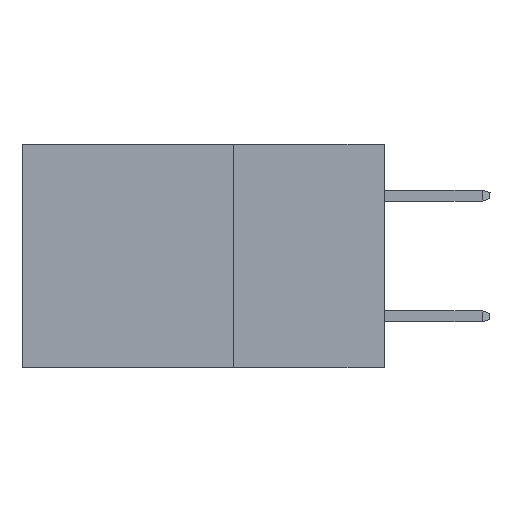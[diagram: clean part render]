
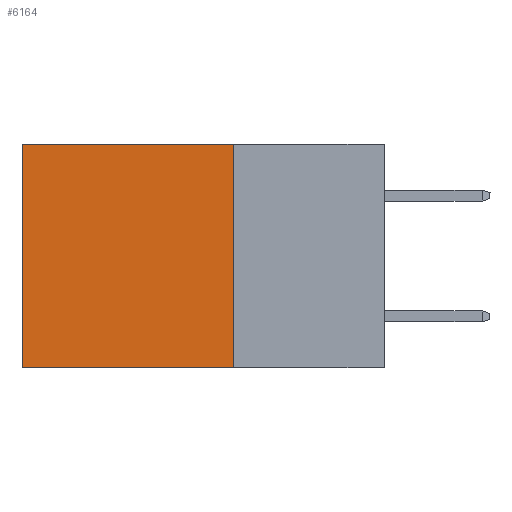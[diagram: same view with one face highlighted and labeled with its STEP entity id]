
A CAD part, left-side view. The second image highlights one B-rep face of the part: STEP entity #6164.
In plain terms, the highlighted planar face has unit normal (-1, 0, 0).
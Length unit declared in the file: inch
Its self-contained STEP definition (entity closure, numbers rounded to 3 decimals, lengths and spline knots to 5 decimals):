
#123 = EDGE_CURVE ( 'NONE', #22109, #328, #17010, .T. ) ;
#328 = VERTEX_POINT ( 'NONE', #18440 ) ;
#465 = DIRECTION ( 'NONE',  ( 0., 0., -1. ) ) ;
#717 = ORIENTED_EDGE ( 'NONE', *, *, #6820, .T. ) ;
#1364 = VERTEX_POINT ( 'NONE', #5905 ) ;
#1472 = EDGE_CURVE ( 'NONE', #1364, #22109, #12091, .T. ) ;
#4559 = ORIENTED_EDGE ( 'NONE', *, *, #123, .F. ) ;
#5905 = CARTESIAN_POINT ( 'NONE',  ( 0.298, 0.25, 0. ) ) ;
#6044 = CARTESIAN_POINT ( 'NONE',  ( 0.298, 0.25, -0.37 ) ) ;
#6164 = ADVANCED_FACE ( 'NONE', ( #22133 ), #16163, .F. ) ;
#6183 = DIRECTION ( 'NONE',  ( 0., 1., 0. ) ) ;
#6373 = DIRECTION ( 'NONE',  ( 0., 0., -1. ) ) ;
#6401 = DIRECTION ( 'NONE',  ( 0., 1., 0. ) ) ;
#6491 = CARTESIAN_POINT ( 'NONE',  ( 0.298, 0.25, 0. ) ) ;
#6820 = EDGE_CURVE ( 'NONE', #1364, #8676, #20206, .T. ) ;
#7930 = EDGE_CURVE ( 'NONE', #8676, #328, #10100, .T. ) ;
#8676 = VERTEX_POINT ( 'NONE', #9246 ) ;
#8745 = VECTOR ( 'NONE', #6373, 39.37008 ) ;
#9246 = CARTESIAN_POINT ( 'NONE',  ( 0.298, 0.6, 0. ) ) ;
#9337 = VECTOR ( 'NONE', #6183, 39.37008 ) ;
#9943 = EDGE_LOOP ( 'NONE', ( #10890, #4559, #16359, #717 ) ) ;
#10100 = LINE ( 'NONE', #16648, #8745 ) ;
#10747 = CARTESIAN_POINT ( 'NONE',  ( 0.298, 0.25, 0. ) ) ;
#10890 = ORIENTED_EDGE ( 'NONE', *, *, #7930, .T. ) ;
#11687 = CARTESIAN_POINT ( 'NONE',  ( 0.298, 0.25, -0.37 ) ) ;
#12091 = LINE ( 'NONE', #10747, #15874 ) ;
#15133 = AXIS2_PLACEMENT_3D ( 'NONE', #16238, #21469, #19592 ) ;
#15874 = VECTOR ( 'NONE', #465, 39.37008 ) ;
#16163 = PLANE ( 'NONE',  #15133 ) ;
#16238 = CARTESIAN_POINT ( 'NONE',  ( 0.298, 0.25, 0. ) ) ;
#16359 = ORIENTED_EDGE ( 'NONE', *, *, #1472, .F. ) ;
#16648 = CARTESIAN_POINT ( 'NONE',  ( 0.298, 0.6, 0. ) ) ;
#17010 = LINE ( 'NONE', #11687, #21104 ) ;
#18440 = CARTESIAN_POINT ( 'NONE',  ( 0.298, 0.6, -0.37 ) ) ;
#19592 = DIRECTION ( 'NONE',  ( 0., 0., -1. ) ) ;
#20206 = LINE ( 'NONE', #6491, #9337 ) ;
#21104 = VECTOR ( 'NONE', #6401, 39.37008 ) ;
#21469 = DIRECTION ( 'NONE',  ( 1., 0., 0. ) ) ;
#22109 = VERTEX_POINT ( 'NONE', #6044 ) ;
#22133 = FACE_OUTER_BOUND ( 'NONE', #9943, .T. ) ;
